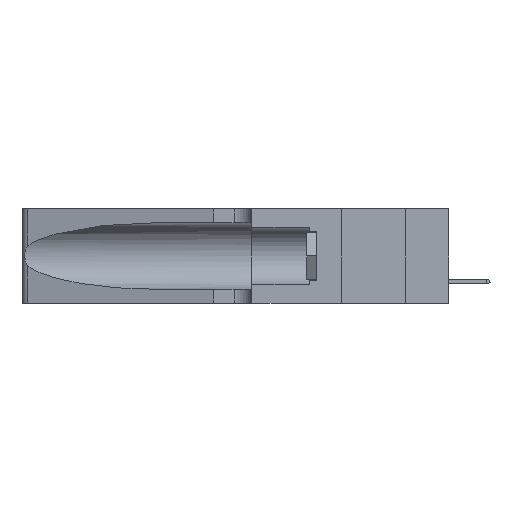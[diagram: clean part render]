
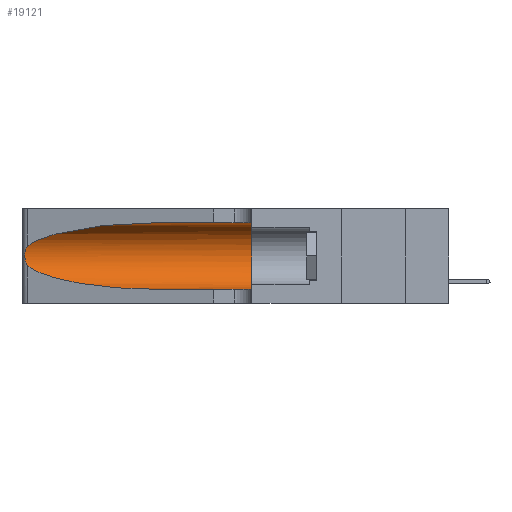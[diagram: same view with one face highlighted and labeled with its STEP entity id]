
A CAD part, left-side view. The second image highlights one B-rep face of the part: STEP entity #19121.
In plain terms, the highlighted cylindrical face has radius 3.308 mm (diameter 6.617 mm), a partial arc.
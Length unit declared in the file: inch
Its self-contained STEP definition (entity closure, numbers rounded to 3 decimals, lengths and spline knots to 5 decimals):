
#1281 = VERTEX_POINT ( 'NONE', #27396 ) ;
#1298 = EDGE_CURVE ( 'NONE', #17045, #25369, #27589, .T. ) ;
#2178 = CARTESIAN_POINT ( 'NONE',  ( 0.25555, 1.22993, 0.14849 ) ) ;
#2937 = VERTEX_POINT ( 'NONE', #23758 ) ;
#4562 = CARTESIAN_POINT ( 'NONE',  ( 0.25555, 1.22994, 0.2215 ) ) ;
#4826 = CARTESIAN_POINT ( 'NONE',  ( 0.25487, 1.22718, 0.22369 ) ) ;
#5166 = AXIS2_PLACEMENT_3D ( 'NONE', #36327, #10311, #16045 ) ;
#5229 = CARTESIAN_POINT ( 'NONE',  ( 0.1305, 0.72297, 0.05475 ) ) ;
#5409 = CARTESIAN_POINT ( 'NONE',  ( 0.26075, 1.23896, 0.178 ) ) ;
#5490 = VECTOR ( 'NONE', #9624, 39.37008 ) ;
#5539 = CARTESIAN_POINT ( 'NONE',  ( 0.25789, 1.23486, 0.15765 ) ) ;
#6125 =( BOUNDED_CURVE ( )  B_SPLINE_CURVE ( 3, ( #24317, #22408, #33534, #5229 ),
 .UNSPECIFIED., .F., .F. ) 
 B_SPLINE_CURVE_WITH_KNOTS ( ( 4, 4 ),
 ( 3.44316, 4.71239 ),
 .UNSPECIFIED. ) 
 CURVE ( )  GEOMETRIC_REPRESENTATION_ITEM ( )  RATIONAL_B_SPLINE_CURVE ( ( 1., 0.87, 0.87, 1. ) ) 
 REPRESENTATION_ITEM ( '' )  );
#6821 = CARTESIAN_POINT ( 'NONE',  ( 0.1305, 0.35, 0.05475 ) ) ;
#8066 = CARTESIAN_POINT ( 'NONE',  ( 0.2373, 1.15595, 0.28018 ) ) ;
#8175 = CARTESIAN_POINT ( 'NONE',  ( 0.25487, 1.22718, 0.14631 ) ) ;
#9152 = LINE ( 'NONE', #22311, #13159 ) ;
#9624 = DIRECTION ( 'NONE',  ( 0., -1., 0. ) ) ;
#10311 = DIRECTION ( 'NONE',  ( 0., -1., 0. ) ) ;
#10415 = DIRECTION ( 'NONE',  ( 0., -1., 0. ) ) ;
#10708 = ORIENTED_EDGE ( 'NONE', *, *, #26554, .T. ) ;
#13159 = VECTOR ( 'NONE', #10415, 39.37008 ) ;
#13779 = CARTESIAN_POINT ( 'NONE',  ( 0.25854, 1.2359, 0.20912 ) ) ;
#14173 = DIRECTION ( 'NONE',  ( 0., 1., 0. ) ) ;
#14872 = ORIENTED_EDGE ( 'NONE', *, *, #1298, .F. ) ;
#15041 = EDGE_CURVE ( 'NONE', #30259, #22824, #36634, .T. ) ;
#15112 = ORIENTED_EDGE ( 'NONE', *, *, #25029, .F. ) ;
#15923 = CARTESIAN_POINT ( 'NONE',  ( 0.25487, 1.22718, 0.22369 ) ) ;
#16045 = DIRECTION ( 'NONE',  ( 0., 0., -1. ) ) ;
#16412 = CARTESIAN_POINT ( 'NONE',  ( 0.26017, 1.23833, 0.17102 ) ) ;
#16654 = CARTESIAN_POINT ( 'NONE',  ( 0.25639, 1.23186, 0.15144 ) ) ;
#17045 = VERTEX_POINT ( 'NONE', #26701 ) ;
#18315 = CYLINDRICAL_SURFACE ( 'NONE', #5166, 0.13025 ) ;
#19121 = ADVANCED_FACE ( 'NONE', ( #22387 ), #18315, .F. ) ;
#19782 = EDGE_CURVE ( 'NONE', #2937, #1281, #6125, .T. ) ;
#20391 = CARTESIAN_POINT ( 'NONE',  ( 0.1305, 1.61858, 0.05475 ) ) ;
#20958 = CARTESIAN_POINT ( 'NONE',  ( 0.25487, 1.22718, 0.22369 ) ) ;
#20990 = EDGE_CURVE ( 'NONE', #22824, #2937, #24524, .T. ) ;
#22073 = LINE ( 'NONE', #20391, #5490 ) ;
#22311 = CARTESIAN_POINT ( 'NONE',  ( 0.1305, 1.61858, 0.31525 ) ) ;
#22387 = FACE_OUTER_BOUND ( 'NONE', #34470, .T. ) ;
#22408 = CARTESIAN_POINT ( 'NONE',  ( 0.2373, 1.15595, 0.08982 ) ) ;
#22796 = ORIENTED_EDGE ( 'NONE', *, *, #19782, .T. ) ;
#22824 = VERTEX_POINT ( 'NONE', #20958 ) ;
#23758 = CARTESIAN_POINT ( 'NONE',  ( 0.25487, 1.22718, 0.14631 ) ) ;
#24317 = CARTESIAN_POINT ( 'NONE',  ( 0.25487, 1.22718, 0.14631 ) ) ;
#24524 = B_SPLINE_CURVE_WITH_KNOTS ( 'NONE', 3,
 ( #15923, #4562, #33581, #30867, #13779, #28476, #33812, #5409, #16412, #28110, #5539, #16654, #2178, #8175 ),
 .UNSPECIFIED., .F., .F.,
 ( 4, 2, 2, 2, 2, 2, 4 ),
 ( 0., 0.00027, 0.00053, 0.00107, 0.0016, 0.00187, 0.00214 ),
 .UNSPECIFIED. ) ;
#25029 = EDGE_CURVE ( 'NONE', #30259, #17045, #9152, .T. ) ;
#25369 = VERTEX_POINT ( 'NONE', #6821 ) ;
#25401 = ORIENTED_EDGE ( 'NONE', *, *, #20990, .T. ) ;
#25506 = CARTESIAN_POINT ( 'NONE',  ( 0.1305, 0.72297, 0.31525 ) ) ;
#26554 = EDGE_CURVE ( 'NONE', #1281, #25369, #22073, .T. ) ;
#26701 = CARTESIAN_POINT ( 'NONE',  ( 0.1305, 0.35, 0.31525 ) ) ;
#27396 = CARTESIAN_POINT ( 'NONE',  ( 0.1305, 0.72297, 0.05475 ) ) ;
#27589 = CIRCLE ( 'NONE', #32511, 0.13025 ) ;
#27629 = CARTESIAN_POINT ( 'NONE',  ( 0.1305, 0.72297, 0.31525 ) ) ;
#28110 = CARTESIAN_POINT ( 'NONE',  ( 0.25856, 1.23593, 0.16098 ) ) ;
#28476 = CARTESIAN_POINT ( 'NONE',  ( 0.26018, 1.23835, 0.19895 ) ) ;
#29282 = ORIENTED_EDGE ( 'NONE', *, *, #15041, .T. ) ;
#30259 = VERTEX_POINT ( 'NONE', #25506 ) ;
#30867 = CARTESIAN_POINT ( 'NONE',  ( 0.25787, 1.23484, 0.2124 ) ) ;
#31390 = CARTESIAN_POINT ( 'NONE',  ( 0.1305, 0.35, 0.185 ) ) ;
#32511 = AXIS2_PLACEMENT_3D ( 'NONE', #31390, #14173, #34728 ) ;
#33474 = CARTESIAN_POINT ( 'NONE',  ( 0.18966, 0.96281, 0.31525 ) ) ;
#33534 = CARTESIAN_POINT ( 'NONE',  ( 0.18966, 0.96281, 0.05475 ) ) ;
#33581 = CARTESIAN_POINT ( 'NONE',  ( 0.25639, 1.23184, 0.21858 ) ) ;
#33812 = CARTESIAN_POINT ( 'NONE',  ( 0.26075, 1.23896, 0.19203 ) ) ;
#34470 = EDGE_LOOP ( 'NONE', ( #29282, #25401, #22796, #10708, #14872, #15112 ) ) ;
#34728 = DIRECTION ( 'NONE',  ( 0., 0., 1. ) ) ;
#36327 = CARTESIAN_POINT ( 'NONE',  ( 0.1305, 1.61858, 0.185 ) ) ;
#36634 =( BOUNDED_CURVE ( )  B_SPLINE_CURVE ( 3, ( #27629, #33474, #8066, #4826 ),
 .UNSPECIFIED., .F., .T. ) 
 B_SPLINE_CURVE_WITH_KNOTS ( ( 4, 4 ),
 ( 1.5708, 2.84003 ),
 .UNSPECIFIED. ) 
 CURVE ( )  GEOMETRIC_REPRESENTATION_ITEM ( )  RATIONAL_B_SPLINE_CURVE ( ( 1., 0.87, 0.87, 1. ) ) 
 REPRESENTATION_ITEM ( '' )  );
